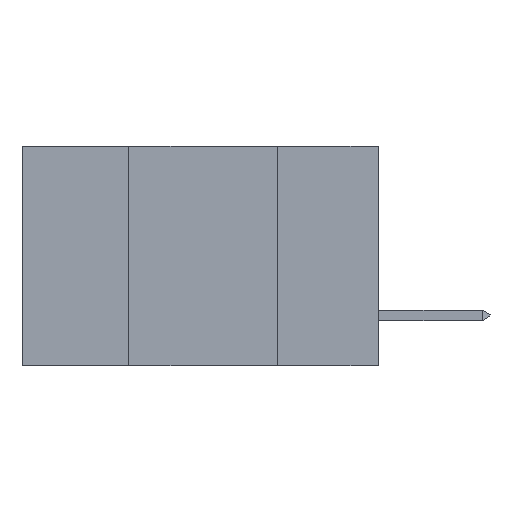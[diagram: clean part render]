
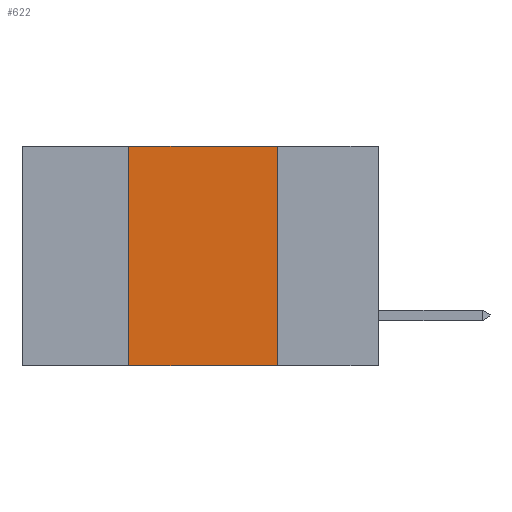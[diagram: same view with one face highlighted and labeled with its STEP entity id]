
A CAD part, left-side view. The second image highlights one B-rep face of the part: STEP entity #622.
In plain terms, the highlighted planar face has unit normal (-1, 0, 0).
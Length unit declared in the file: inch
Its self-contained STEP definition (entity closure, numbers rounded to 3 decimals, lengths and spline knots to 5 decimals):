
#622 = ADVANCED_FACE ( 'NONE', ( #3129 ), #3969, .F. ) ;
#638 = LINE ( 'NONE', #3401, #8763 ) ;
#1138 = ORIENTED_EDGE ( 'NONE', *, *, #7894, .T. ) ;
#1193 = CARTESIAN_POINT ( 'NONE',  ( 0., 0.17, -0.37 ) ) ;
#1239 = VECTOR ( 'NONE', #4848, 39.37008 ) ;
#2320 = VERTEX_POINT ( 'NONE', #2349 ) ;
#2349 = CARTESIAN_POINT ( 'NONE',  ( 0., 0.17, 0. ) ) ;
#2448 = DIRECTION ( 'NONE',  ( 0., 0., 1. ) ) ;
#2853 = DIRECTION ( 'NONE',  ( 0., -1., 0. ) ) ;
#3038 = DIRECTION ( 'NONE',  ( 0., 0., -1. ) ) ;
#3129 = FACE_OUTER_BOUND ( 'NONE', #6896, .T. ) ;
#3187 = DIRECTION ( 'NONE',  ( 1., 0., 0. ) ) ;
#3401 = CARTESIAN_POINT ( 'NONE',  ( 0., 0.6, 0. ) ) ;
#3446 = ORIENTED_EDGE ( 'NONE', *, *, #4850, .F. ) ;
#3528 = LINE ( 'NONE', #9474, #7797 ) ;
#3969 = PLANE ( 'NONE',  #8346 ) ;
#4696 = VERTEX_POINT ( 'NONE', #7585 ) ;
#4848 = DIRECTION ( 'NONE',  ( 0., 0., -1. ) ) ;
#4850 = EDGE_CURVE ( 'NONE', #4696, #7843, #7643, .T. ) ;
#5603 = ORIENTED_EDGE ( 'NONE', *, *, #6129, .F. ) ;
#6129 = EDGE_CURVE ( 'NONE', #2320, #6944, #6922, .T. ) ;
#6479 = DIRECTION ( 'NONE',  ( 0., -1., 0. ) ) ;
#6654 = CARTESIAN_POINT ( 'NONE',  ( 0., 0.42, 0. ) ) ;
#6682 = EDGE_CURVE ( 'NONE', #7843, #2320, #638, .T. ) ;
#6896 = EDGE_LOOP ( 'NONE', ( #5603, #9250, #3446, #1138 ) ) ;
#6922 = LINE ( 'NONE', #1193, #1239 ) ;
#6944 = VERTEX_POINT ( 'NONE', #8511 ) ;
#7234 = VECTOR ( 'NONE', #2448, 39.37008 ) ;
#7585 = CARTESIAN_POINT ( 'NONE',  ( 0., 0.42, -0.37 ) ) ;
#7643 = LINE ( 'NONE', #9225, #7234 ) ;
#7797 = VECTOR ( 'NONE', #2853, 39.37008 ) ;
#7843 = VERTEX_POINT ( 'NONE', #6654 ) ;
#7894 = EDGE_CURVE ( 'NONE', #4696, #6944, #3528, .T. ) ;
#8293 = CARTESIAN_POINT ( 'NONE',  ( 0., 0.6, 0. ) ) ;
#8346 = AXIS2_PLACEMENT_3D ( 'NONE', #8293, #3187, #3038 ) ;
#8511 = CARTESIAN_POINT ( 'NONE',  ( 0., 0.17, -0.37 ) ) ;
#8763 = VECTOR ( 'NONE', #6479, 39.37008 ) ;
#9225 = CARTESIAN_POINT ( 'NONE',  ( 0., 0.42, -0.37 ) ) ;
#9250 = ORIENTED_EDGE ( 'NONE', *, *, #6682, .F. ) ;
#9474 = CARTESIAN_POINT ( 'NONE',  ( 0., 0.6, -0.37 ) ) ;
